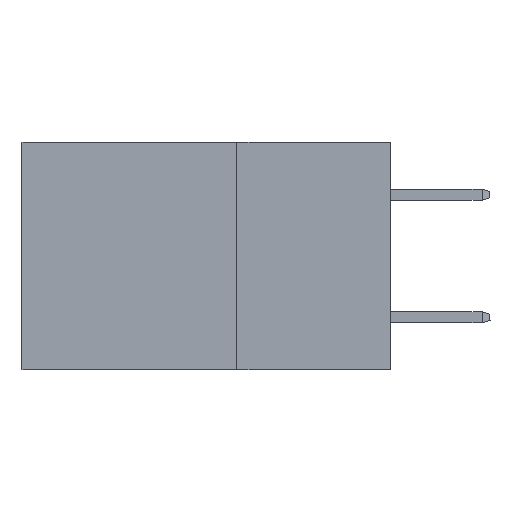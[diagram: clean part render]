
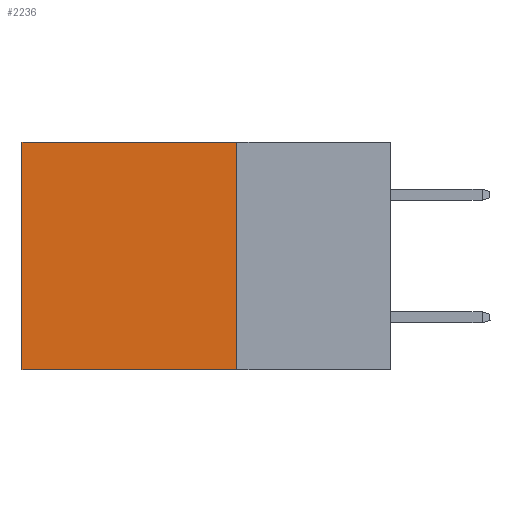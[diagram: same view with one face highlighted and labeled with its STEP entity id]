
A CAD part, left-side view. The second image highlights one B-rep face of the part: STEP entity #2236.
In plain terms, the highlighted planar face has unit normal (-1, 0, 0).
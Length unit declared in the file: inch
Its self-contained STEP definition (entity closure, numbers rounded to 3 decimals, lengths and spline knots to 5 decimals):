
#1291 = LINE ( 'NONE', #13937, #19693 ) ;
#2236 = ADVANCED_FACE ( 'NONE', ( #5056 ), #5489, .F. ) ;
#3032 = LINE ( 'NONE', #6223, #15461 ) ;
#3163 = LINE ( 'NONE', #15772, #20916 ) ;
#4373 = ORIENTED_EDGE ( 'NONE', *, *, #23356, .T. ) ;
#5056 = FACE_OUTER_BOUND ( 'NONE', #6814, .T. ) ;
#5489 = PLANE ( 'NONE',  #15204 ) ;
#5845 = ORIENTED_EDGE ( 'NONE', *, *, #18334, .F. ) ;
#6113 = EDGE_CURVE ( 'NONE', #7378, #9918, #3163, .T. ) ;
#6223 = CARTESIAN_POINT ( 'NONE',  ( 0.2875, 0.25, 0. ) ) ;
#6814 = EDGE_LOOP ( 'NONE', ( #9563, #18855, #5845, #4373 ) ) ;
#6973 = LINE ( 'NONE', #10827, #14178 ) ;
#7378 = VERTEX_POINT ( 'NONE', #16488 ) ;
#8862 = DIRECTION ( 'NONE',  ( 0., 0., -1. ) ) ;
#9221 = DIRECTION ( 'NONE',  ( 0., 0., -1. ) ) ;
#9563 = ORIENTED_EDGE ( 'NONE', *, *, #24561, .T. ) ;
#9898 = CARTESIAN_POINT ( 'NONE',  ( 0.2875, 0.25, 0. ) ) ;
#9918 = VERTEX_POINT ( 'NONE', #16083 ) ;
#10827 = CARTESIAN_POINT ( 'NONE',  ( 0.2875, 0.6, 0. ) ) ;
#13937 = CARTESIAN_POINT ( 'NONE',  ( 0.2875, 0.25, 0. ) ) ;
#14178 = VECTOR ( 'NONE', #8862, 39.37008 ) ;
#14286 = VERTEX_POINT ( 'NONE', #21577 ) ;
#14901 = CARTESIAN_POINT ( 'NONE',  ( 0.2875, 0.25, 0. ) ) ;
#15204 = AXIS2_PLACEMENT_3D ( 'NONE', #14901, #24560, #9221 ) ;
#15461 = VECTOR ( 'NONE', #19782, 39.37008 ) ;
#15772 = CARTESIAN_POINT ( 'NONE',  ( 0.2875, 0.25, -0.37 ) ) ;
#16083 = CARTESIAN_POINT ( 'NONE',  ( 0.2875, 0.6, -0.37 ) ) ;
#16488 = CARTESIAN_POINT ( 'NONE',  ( 0.2875, 0.25, -0.37 ) ) ;
#18334 = EDGE_CURVE ( 'NONE', #19938, #7378, #3032, .T. ) ;
#18855 = ORIENTED_EDGE ( 'NONE', *, *, #6113, .F. ) ;
#19693 = VECTOR ( 'NONE', #21307, 39.37008 ) ;
#19782 = DIRECTION ( 'NONE',  ( 0., 0., -1. ) ) ;
#19938 = VERTEX_POINT ( 'NONE', #9898 ) ;
#20916 = VECTOR ( 'NONE', #23573, 39.37008 ) ;
#21307 = DIRECTION ( 'NONE',  ( 0., 1., 0. ) ) ;
#21577 = CARTESIAN_POINT ( 'NONE',  ( 0.2875, 0.6, 0. ) ) ;
#23356 = EDGE_CURVE ( 'NONE', #19938, #14286, #1291, .T. ) ;
#23573 = DIRECTION ( 'NONE',  ( 0., 1., 0. ) ) ;
#24560 = DIRECTION ( 'NONE',  ( 1., 0., 0. ) ) ;
#24561 = EDGE_CURVE ( 'NONE', #14286, #9918, #6973, .T. ) ;
